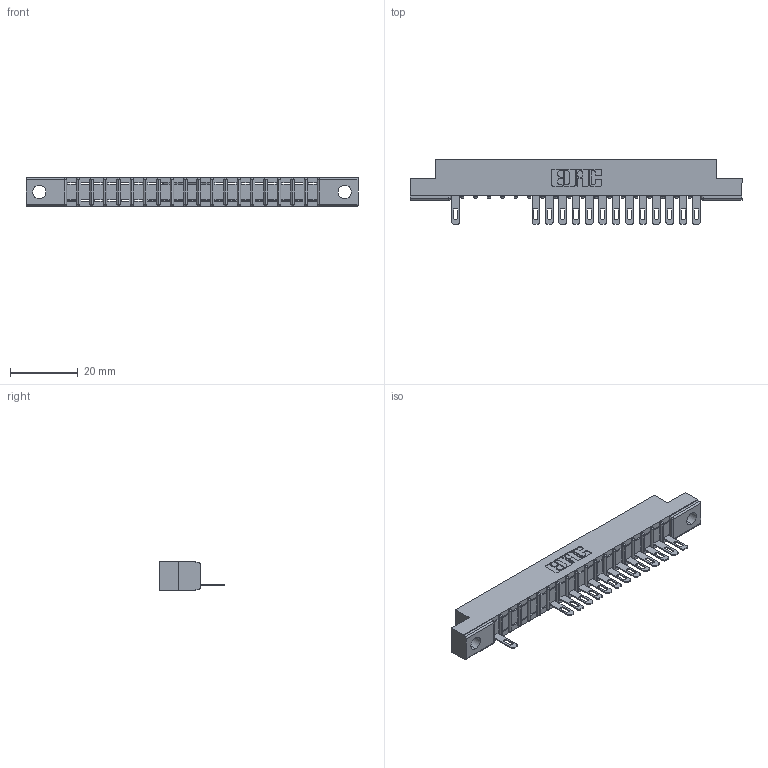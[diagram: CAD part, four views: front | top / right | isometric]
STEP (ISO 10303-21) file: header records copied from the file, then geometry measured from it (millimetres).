
FILE_DESCRIPTION (( 'STEP AP203' ), '1' );
FILE_NAME ('357-019-505-104.STEP', '2018-08-08T06:06:14', ( '' ), ( '' ), 'SwSTEP 2.0', 'SolidWorks 2016', '' );
FILE_SCHEMA (( 'CONFIG_CONTROL_DESIGN' ));
Length unit declared in the file: inch
Products named in the file (3): 307 Part_.156 Dia Mounting Holes; 307-290-001_505; 357-019-505-104
Assembly tree (15 placements, depth 2):
  357-019-505-104
    307 Part_.156 Dia Mounting Holes
    307-290-001_505  x14
Bounding box: 98.3 x 19.18 x 8.71 mm (x, y, z)
Volume: 222 mm3; surface area: 8826.2 mm2
Topology: 14 solids, 15 shells, 1036 faces, 2946 edges, 1890 vertices
Faces by surface type: plane 648, cylinder 348, sphere 40
Entity records: 19356 total; most frequent: CARTESIAN_POINT 3277, ORIENTED_EDGE 3266, DIRECTION 3189, EDGE_CURVE 1633, LINE 1249, VECTOR 1249, VERTEX_POINT 1058, AXIS2_PLACEMENT_3D 970
